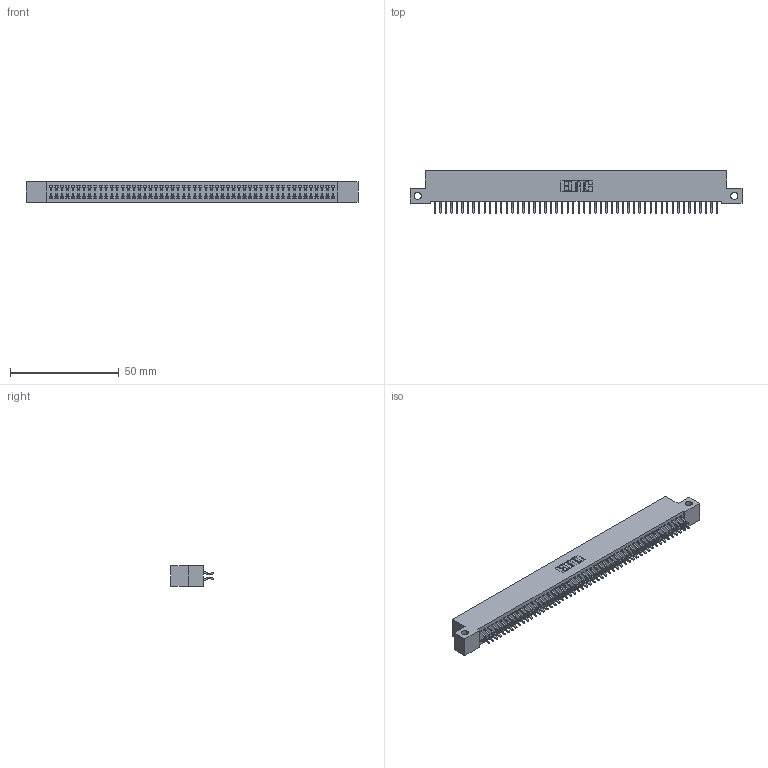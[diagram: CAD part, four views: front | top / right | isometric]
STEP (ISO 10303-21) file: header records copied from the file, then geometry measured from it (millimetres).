
FILE_DESCRIPTION (( 'STEP AP203' ), '1' );
FILE_NAME ('392-104-556-212.STEP', '2018-08-18T19:51:01', ( '' ), ( '' ), 'SwSTEP 2.0', 'SolidWorks 2016', '' );
FILE_SCHEMA (( 'CONFIG_CONTROL_DESIGN' ));
Length unit declared in the file: inch
Products named in the file (3): 342 Part_Side Mount; 345-292-001_556 Tail; 392-104-556-212
Assembly tree (105 placements, depth 2):
  392-104-556-212
    342 Part_Side Mount
    345-292-001_556 Tail  x104
Bounding box: 152.4 x 19.58 x 9.4 mm (x, y, z)
Volume: 13663.9 mm3; surface area: 22227.1 mm2
Topology: 105 solids, 105 shells, 6142 faces, 18291 edges, 12054 vertices
Faces by surface type: plane 4226, cylinder 1916
Entity records: 32251 total; most frequent: CARTESIAN_POINT 5346, ORIENTED_EDGE 5270, DIRECTION 4539, EDGE_CURVE 2635, VECTOR 2499, LINE 2499, VERTEX_POINT 1754, AXIS2_PLACEMENT_3D 1020
